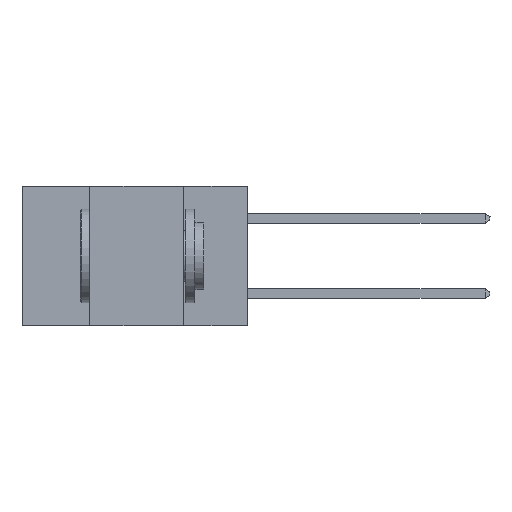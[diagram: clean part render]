
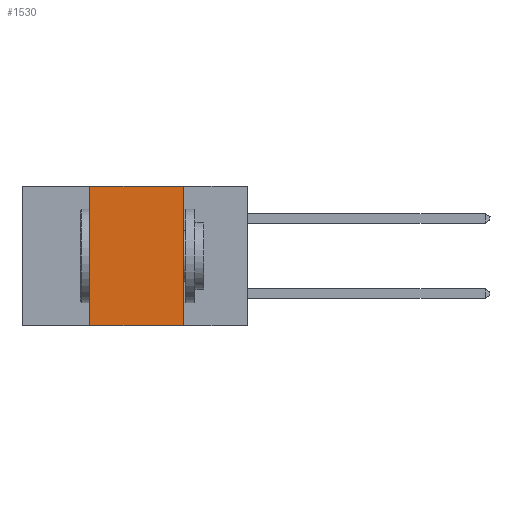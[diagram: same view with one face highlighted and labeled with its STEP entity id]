
A CAD part, left-side view. The second image highlights one B-rep face of the part: STEP entity #1530.
In plain terms, the highlighted planar face has unit normal (-1, 0, 0).
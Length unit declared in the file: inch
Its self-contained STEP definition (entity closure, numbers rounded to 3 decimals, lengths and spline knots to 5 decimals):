
#161 = DIRECTION ( 'NONE',  ( 1., 0., 0. ) ) ;
#166 = DIRECTION ( 'NONE',  ( 0., 0., -1. ) ) ;
#304 = LINE ( 'NONE', #12945, #10959 ) ;
#769 = VERTEX_POINT ( 'NONE', #4907 ) ;
#1150 = VERTEX_POINT ( 'NONE', #12633 ) ;
#1530 = ADVANCED_FACE ( 'NONE', ( #7329 ), #5329, .F. ) ;
#2148 = EDGE_CURVE ( 'NONE', #1150, #769, #2337, .T. ) ;
#2337 = LINE ( 'NONE', #11429, #2485 ) ;
#2485 = VECTOR ( 'NONE', #166, 39.37008 ) ;
#2745 = DIRECTION ( 'NONE',  ( 0., -1., 0. ) ) ;
#2898 = EDGE_CURVE ( 'NONE', #8987, #1150, #12060, .T. ) ;
#2984 = DIRECTION ( 'NONE',  ( 0., -1., 0. ) ) ;
#4154 = DIRECTION ( 'NONE',  ( 0., 0., -1. ) ) ;
#4221 = EDGE_CURVE ( 'NONE', #13230, #8987, #4588, .T. ) ;
#4369 = ORIENTED_EDGE ( 'NONE', *, *, #12289, .T. ) ;
#4588 = LINE ( 'NONE', #5702, #6703 ) ;
#4907 = CARTESIAN_POINT ( 'NONE',  ( 0., 0.17, -0.37 ) ) ;
#5139 = CARTESIAN_POINT ( 'NONE',  ( 0., 0.6, 0. ) ) ;
#5305 = CARTESIAN_POINT ( 'NONE',  ( 0., 0.42, -0.37 ) ) ;
#5329 = PLANE ( 'NONE',  #8095 ) ;
#5702 = CARTESIAN_POINT ( 'NONE',  ( 0., 0.42, 0. ) ) ;
#6429 = VECTOR ( 'NONE', #2984, 39.37008 ) ;
#6667 = ORIENTED_EDGE ( 'NONE', *, *, #2148, .F. ) ;
#6703 = VECTOR ( 'NONE', #8825, 39.37008 ) ;
#7329 = FACE_OUTER_BOUND ( 'NONE', #10953, .T. ) ;
#8095 = AXIS2_PLACEMENT_3D ( 'NONE', #9377, #161, #4154 ) ;
#8404 = ORIENTED_EDGE ( 'NONE', *, *, #2898, .F. ) ;
#8645 = ORIENTED_EDGE ( 'NONE', *, *, #4221, .F. ) ;
#8664 = CARTESIAN_POINT ( 'NONE',  ( 0., 0.42, 0. ) ) ;
#8825 = DIRECTION ( 'NONE',  ( 0., 0., 1. ) ) ;
#8987 = VERTEX_POINT ( 'NONE', #8664 ) ;
#9377 = CARTESIAN_POINT ( 'NONE',  ( 0., 0.6, 0. ) ) ;
#10953 = EDGE_LOOP ( 'NONE', ( #6667, #8404, #8645, #4369 ) ) ;
#10959 = VECTOR ( 'NONE', #2745, 39.37008 ) ;
#11429 = CARTESIAN_POINT ( 'NONE',  ( 0., 0.17, 0. ) ) ;
#12060 = LINE ( 'NONE', #5139, #6429 ) ;
#12289 = EDGE_CURVE ( 'NONE', #13230, #769, #304, .T. ) ;
#12633 = CARTESIAN_POINT ( 'NONE',  ( 0., 0.17, 0. ) ) ;
#12945 = CARTESIAN_POINT ( 'NONE',  ( 0., 0.6, -0.37 ) ) ;
#13230 = VERTEX_POINT ( 'NONE', #5305 ) ;
